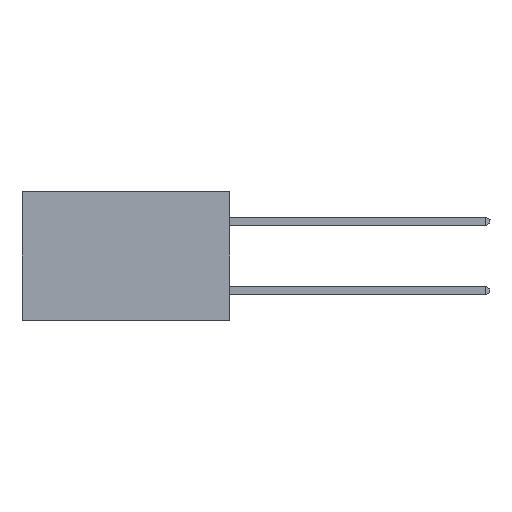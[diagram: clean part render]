
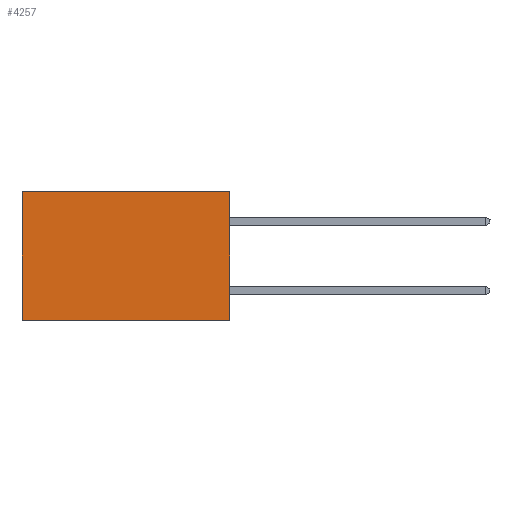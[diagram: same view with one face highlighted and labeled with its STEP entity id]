
A CAD part, left-side view. The second image highlights one B-rep face of the part: STEP entity #4257.
In plain terms, the highlighted planar face has unit normal (-1, 0, 0).
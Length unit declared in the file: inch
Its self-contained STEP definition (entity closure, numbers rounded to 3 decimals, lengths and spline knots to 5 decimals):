
#344 = VERTEX_POINT ( 'NONE', #2267 ) ;
#478 = DIRECTION ( 'NONE',  ( 0., 1., 0. ) ) ;
#605 = ORIENTED_EDGE ( 'NONE', *, *, #5165, .T. ) ;
#641 = ORIENTED_EDGE ( 'NONE', *, *, #5650, .F. ) ;
#888 = CARTESIAN_POINT ( 'NONE',  ( 0.298, 0., 0. ) ) ;
#915 = LINE ( 'NONE', #2166, #8613 ) ;
#947 = CARTESIAN_POINT ( 'NONE',  ( 0.298, 0., 0. ) ) ;
#1358 = DIRECTION ( 'NONE',  ( 0., 0., -1. ) ) ;
#1484 = ORIENTED_EDGE ( 'NONE', *, *, #5849, .F. ) ;
#1858 = VERTEX_POINT ( 'NONE', #3497 ) ;
#2166 = CARTESIAN_POINT ( 'NONE',  ( 0.298, 0., -0.37 ) ) ;
#2167 = VECTOR ( 'NONE', #9894, 39.37008 ) ;
#2267 = CARTESIAN_POINT ( 'NONE',  ( 0.298, 0., -0.37 ) ) ;
#2580 = LINE ( 'NONE', #888, #5709 ) ;
#3497 = CARTESIAN_POINT ( 'NONE',  ( 0.298, 0.6, 0. ) ) ;
#3643 = LINE ( 'NONE', #9821, #2167 ) ;
#4257 = ADVANCED_FACE ( 'NONE', ( #7766 ), #5619, .F. ) ;
#4470 = ORIENTED_EDGE ( 'NONE', *, *, #10540, .T. ) ;
#4589 = AXIS2_PLACEMENT_3D ( 'NONE', #8977, #9091, #1358 ) ;
#4690 = VECTOR ( 'NONE', #9239, 39.37008 ) ;
#5165 = EDGE_CURVE ( 'NONE', #1858, #5488, #9162, .T. ) ;
#5488 = VERTEX_POINT ( 'NONE', #8958 ) ;
#5619 = PLANE ( 'NONE',  #4589 ) ;
#5650 = EDGE_CURVE ( 'NONE', #344, #5488, #915, .T. ) ;
#5709 = VECTOR ( 'NONE', #7733, 39.37008 ) ;
#5849 = EDGE_CURVE ( 'NONE', #10799, #344, #2580, .T. ) ;
#7732 = EDGE_LOOP ( 'NONE', ( #605, #641, #1484, #4470 ) ) ;
#7733 = DIRECTION ( 'NONE',  ( 0., 0., -1. ) ) ;
#7766 = FACE_OUTER_BOUND ( 'NONE', #7732, .T. ) ;
#8613 = VECTOR ( 'NONE', #478, 39.37008 ) ;
#8958 = CARTESIAN_POINT ( 'NONE',  ( 0.298, 0.6, -0.37 ) ) ;
#8977 = CARTESIAN_POINT ( 'NONE',  ( 0.298, 0., 0. ) ) ;
#9091 = DIRECTION ( 'NONE',  ( 1., 0., 0. ) ) ;
#9162 = LINE ( 'NONE', #10866, #4690 ) ;
#9239 = DIRECTION ( 'NONE',  ( 0., 0., -1. ) ) ;
#9821 = CARTESIAN_POINT ( 'NONE',  ( 0.298, 0., 0. ) ) ;
#9894 = DIRECTION ( 'NONE',  ( 0., 1., 0. ) ) ;
#10540 = EDGE_CURVE ( 'NONE', #10799, #1858, #3643, .T. ) ;
#10799 = VERTEX_POINT ( 'NONE', #947 ) ;
#10866 = CARTESIAN_POINT ( 'NONE',  ( 0.298, 0.6, 0. ) ) ;
